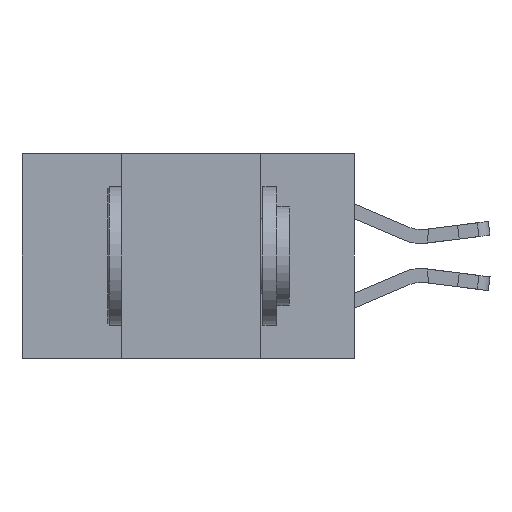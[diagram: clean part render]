
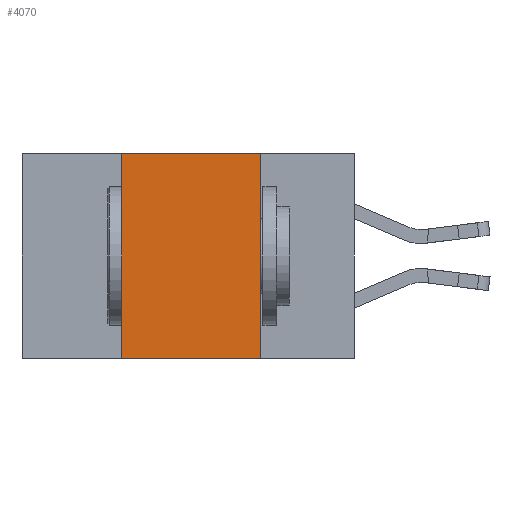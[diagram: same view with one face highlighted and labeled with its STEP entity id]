
A CAD part, left-side view. The second image highlights one B-rep face of the part: STEP entity #4070.
In plain terms, the highlighted planar face has unit normal (-1, 0, 0).
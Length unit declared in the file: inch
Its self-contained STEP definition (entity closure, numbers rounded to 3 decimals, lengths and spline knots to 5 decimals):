
#425 = CARTESIAN_POINT ( 'NONE',  ( 0., 0.17, -0.37 ) ) ;
#592 = CARTESIAN_POINT ( 'NONE',  ( 0., 0.42, -0.37 ) ) ;
#683 = CARTESIAN_POINT ( 'NONE',  ( 0., 0.42, 0. ) ) ;
#736 = VECTOR ( 'NONE', #8108, 39.37008 ) ;
#869 = VERTEX_POINT ( 'NONE', #6685 ) ;
#1268 = VECTOR ( 'NONE', #10702, 39.37008 ) ;
#2083 = LINE ( 'NONE', #9003, #12438 ) ;
#3510 = CARTESIAN_POINT ( 'NONE',  ( 0., 0.6, 0. ) ) ;
#3527 = DIRECTION ( 'NONE',  ( 0., -1., 0. ) ) ;
#3685 = VERTEX_POINT ( 'NONE', #683 ) ;
#4070 = ADVANCED_FACE ( 'NONE', ( #6120 ), #10118, .F. ) ;
#4179 = LINE ( 'NONE', #9589, #1268 ) ;
#4612 = DIRECTION ( 'NONE',  ( 0., 0., -1. ) ) ;
#4973 = CARTESIAN_POINT ( 'NONE',  ( 0., 0.17, -0.37 ) ) ;
#6120 = FACE_OUTER_BOUND ( 'NONE', #6482, .T. ) ;
#6482 = EDGE_LOOP ( 'NONE', ( #11674, #11936, #8839, #11713 ) ) ;
#6571 = LINE ( 'NONE', #425, #736 ) ;
#6685 = CARTESIAN_POINT ( 'NONE',  ( 0., 0.17, 0. ) ) ;
#7105 = EDGE_CURVE ( 'NONE', #869, #14063, #6571, .T. ) ;
#7292 = CARTESIAN_POINT ( 'NONE',  ( 0., 0.42, -0.37 ) ) ;
#7422 = AXIS2_PLACEMENT_3D ( 'NONE', #3510, #11228, #4612 ) ;
#7437 = VECTOR ( 'NONE', #13911, 39.37008 ) ;
#7878 = EDGE_CURVE ( 'NONE', #10436, #3685, #13668, .T. ) ;
#8108 = DIRECTION ( 'NONE',  ( 0., 0., -1. ) ) ;
#8519 = EDGE_CURVE ( 'NONE', #10436, #14063, #4179, .T. ) ;
#8839 = ORIENTED_EDGE ( 'NONE', *, *, #7878, .F. ) ;
#9003 = CARTESIAN_POINT ( 'NONE',  ( 0., 0.6, 0. ) ) ;
#9589 = CARTESIAN_POINT ( 'NONE',  ( 0., 0.6, -0.37 ) ) ;
#10118 = PLANE ( 'NONE',  #7422 ) ;
#10190 = EDGE_CURVE ( 'NONE', #3685, #869, #2083, .T. ) ;
#10436 = VERTEX_POINT ( 'NONE', #592 ) ;
#10702 = DIRECTION ( 'NONE',  ( 0., -1., 0. ) ) ;
#11228 = DIRECTION ( 'NONE',  ( 1., 0., 0. ) ) ;
#11674 = ORIENTED_EDGE ( 'NONE', *, *, #7105, .F. ) ;
#11713 = ORIENTED_EDGE ( 'NONE', *, *, #8519, .T. ) ;
#11936 = ORIENTED_EDGE ( 'NONE', *, *, #10190, .F. ) ;
#12438 = VECTOR ( 'NONE', #3527, 39.37008 ) ;
#13668 = LINE ( 'NONE', #7292, #7437 ) ;
#13911 = DIRECTION ( 'NONE',  ( 0., 0., 1. ) ) ;
#14063 = VERTEX_POINT ( 'NONE', #4973 ) ;
